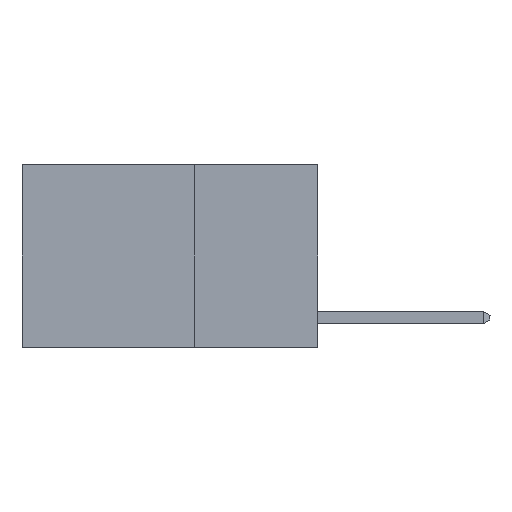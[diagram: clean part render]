
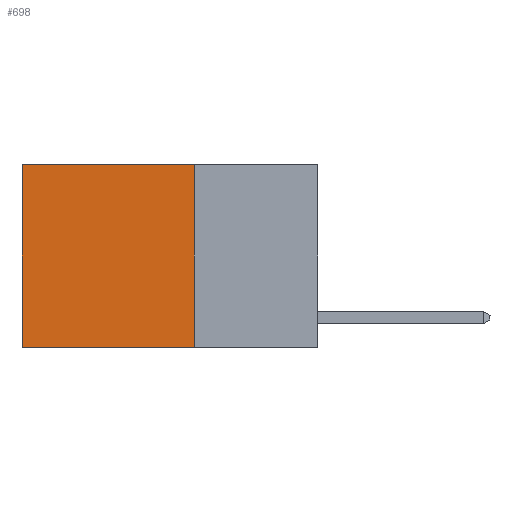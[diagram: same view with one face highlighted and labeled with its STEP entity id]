
A CAD part, left-side view. The second image highlights one B-rep face of the part: STEP entity #698.
In plain terms, the highlighted planar face has unit normal (-1, 0, 0).
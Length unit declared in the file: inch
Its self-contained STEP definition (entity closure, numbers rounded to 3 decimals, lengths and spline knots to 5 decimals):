
#270 = ORIENTED_EDGE ( 'NONE', *, *, #27441, .F. ) ;
#602 = EDGE_LOOP ( 'NONE', ( #13886, #270, #19659, #16097 ) ) ;
#605 = CARTESIAN_POINT ( 'NONE',  ( 0.2625, 0.6, 0. ) ) ;
#698 = ADVANCED_FACE ( 'NONE', ( #10798 ), #23187, .F. ) ;
#1147 = VERTEX_POINT ( 'NONE', #4605 ) ;
#1416 = LINE ( 'NONE', #18630, #12752 ) ;
#1538 = DIRECTION ( 'NONE',  ( 0., 0., -1. ) ) ;
#1834 = VECTOR ( 'NONE', #1538, 39.37008 ) ;
#2871 = DIRECTION ( 'NONE',  ( 0., 0., -1. ) ) ;
#2925 = EDGE_CURVE ( 'NONE', #6554, #1147, #10354, .T. ) ;
#3045 = CARTESIAN_POINT ( 'NONE',  ( 0.2625, 0.25, 0. ) ) ;
#3208 = CARTESIAN_POINT ( 'NONE',  ( 0.2625, 0.6, -0.37 ) ) ;
#4605 = CARTESIAN_POINT ( 'NONE',  ( 0.2625, 0.6, 0. ) ) ;
#4742 = EDGE_CURVE ( 'NONE', #6554, #14922, #25675, .T. ) ;
#6554 = VERTEX_POINT ( 'NONE', #19266 ) ;
#6609 = CARTESIAN_POINT ( 'NONE',  ( 0.2625, 0.25, 0. ) ) ;
#7623 = AXIS2_PLACEMENT_3D ( 'NONE', #3045, #9920, #25487 ) ;
#9920 = DIRECTION ( 'NONE',  ( 1., 0., 0. ) ) ;
#10354 = LINE ( 'NONE', #6609, #28074 ) ;
#10483 = VERTEX_POINT ( 'NONE', #3208 ) ;
#10798 = FACE_OUTER_BOUND ( 'NONE', #602, .T. ) ;
#12752 = VECTOR ( 'NONE', #20830, 39.37008 ) ;
#13886 = ORIENTED_EDGE ( 'NONE', *, *, #20846, .T. ) ;
#14922 = VERTEX_POINT ( 'NONE', #20865 ) ;
#15589 = DIRECTION ( 'NONE',  ( 0., 1., 0. ) ) ;
#16097 = ORIENTED_EDGE ( 'NONE', *, *, #2925, .T. ) ;
#17280 = CARTESIAN_POINT ( 'NONE',  ( 0.2625, 0.25, 0. ) ) ;
#17610 = VECTOR ( 'NONE', #2871, 39.37008 ) ;
#18630 = CARTESIAN_POINT ( 'NONE',  ( 0.2625, 0.25, -0.37 ) ) ;
#19266 = CARTESIAN_POINT ( 'NONE',  ( 0.2625, 0.25, 0. ) ) ;
#19659 = ORIENTED_EDGE ( 'NONE', *, *, #4742, .F. ) ;
#20830 = DIRECTION ( 'NONE',  ( 0., 1., 0. ) ) ;
#20846 = EDGE_CURVE ( 'NONE', #1147, #10483, #24183, .T. ) ;
#20865 = CARTESIAN_POINT ( 'NONE',  ( 0.2625, 0.25, -0.37 ) ) ;
#23187 = PLANE ( 'NONE',  #7623 ) ;
#24183 = LINE ( 'NONE', #605, #17610 ) ;
#25487 = DIRECTION ( 'NONE',  ( 0., 0., -1. ) ) ;
#25675 = LINE ( 'NONE', #17280, #1834 ) ;
#27441 = EDGE_CURVE ( 'NONE', #14922, #10483, #1416, .T. ) ;
#28074 = VECTOR ( 'NONE', #15589, 39.37008 ) ;
